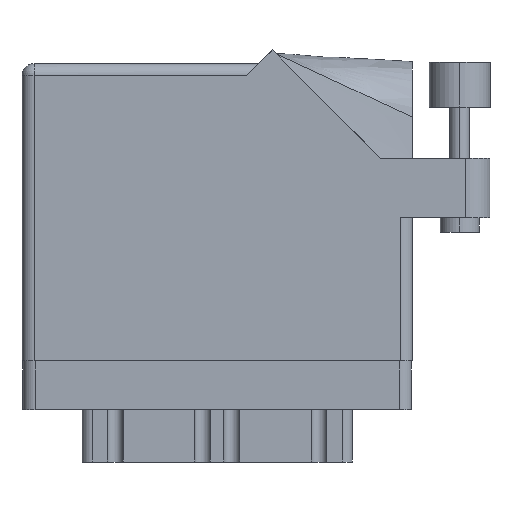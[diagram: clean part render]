
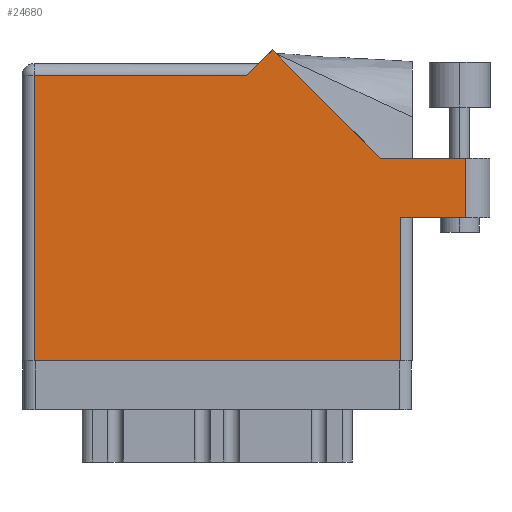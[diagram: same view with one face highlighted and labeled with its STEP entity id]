
A CAD part, front view. The second image highlights one B-rep face of the part: STEP entity #24680.
In plain terms, the highlighted face is planar.
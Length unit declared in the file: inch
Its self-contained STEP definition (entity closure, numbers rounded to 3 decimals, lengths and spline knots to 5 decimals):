
#1559 = ORIENTED_EDGE ( 'NONE', *, *, #2571, .T. ) ;
#2333 = ORIENTED_EDGE ( 'NONE', *, *, #17086, .T. ) ;
#2571 = EDGE_CURVE ( 'NONE', #23713, #5768, #15091, .T. ) ;
#3127 = CARTESIAN_POINT ( 'NONE',  ( 0., 0., 0. ) ) ;
#3396 = EDGE_CURVE ( 'NONE', #16580, #17443, #18091, .T. ) ;
#3887 = VERTEX_POINT ( 'NONE', #12152 ) ;
#4349 = VERTEX_POINT ( 'NONE', #8988 ) ;
#4806 = VECTOR ( 'NONE', #21428, 39.37008 ) ;
#4832 = DIRECTION ( 'NONE',  ( -0.707, -0.707, 0. ) ) ;
#4907 = VECTOR ( 'NONE', #36426, 39.37008 ) ;
#4942 = CARTESIAN_POINT ( 'NONE',  ( 1.948, 0.737, 0. ) ) ;
#5768 = VERTEX_POINT ( 'NONE', #22979 ) ;
#5794 = VECTOR ( 'NONE', #35660, 39.37008 ) ;
#6322 = CARTESIAN_POINT ( 'NONE',  ( 1.84442, 1.044, 0. ) ) ;
#6960 = VECTOR ( 'NONE', #11579, 39.37008 ) ;
#7881 = LINE ( 'NONE', #4942, #11786 ) ;
#8988 = CARTESIAN_POINT ( 'NONE',  ( 0.062, 0., 0. ) ) ;
#9428 = ORIENTED_EDGE ( 'NONE', *, *, #17477, .T. ) ;
#9604 = LINE ( 'NONE', #10342, #4907 ) ;
#9712 = CARTESIAN_POINT ( 'NONE',  ( 1.28771, 1.60071, 0. ) ) ;
#9888 = LINE ( 'NONE', #21854, #22098 ) ;
#10342 = CARTESIAN_POINT ( 'NONE',  ( 2.41, 1.044, 0. ) ) ;
#10674 = CARTESIAN_POINT ( 'NONE',  ( 2.285, 0.737, 0. ) ) ;
#10736 = CARTESIAN_POINT ( 'NONE',  ( 1.217, 1.53, 0. ) ) ;
#10781 = DIRECTION ( 'NONE',  ( 0., 0., -1. ) ) ;
#11579 = DIRECTION ( 'NONE',  ( 0., -1., 0. ) ) ;
#11753 = CARTESIAN_POINT ( 'NONE',  ( 2.285, 1.044, 0. ) ) ;
#11786 = VECTOR ( 'NONE', #23551, 39.37008 ) ;
#12051 = CARTESIAN_POINT ( 'NONE',  ( 1.155, 1.468, 0. ) ) ;
#12087 = ORIENTED_EDGE ( 'NONE', *, *, #24741, .T. ) ;
#12152 = CARTESIAN_POINT ( 'NONE',  ( 1.948, 0.737, 0. ) ) ;
#13011 = DIRECTION ( 'NONE',  ( 1., 0., 0. ) ) ;
#13699 = PLANE ( 'NONE',  #29612 ) ;
#13916 = EDGE_LOOP ( 'NONE', ( #12087, #1559, #15913, #26260, #2333, #9428, #22366, #23523, #27775 ) ) ;
#14127 = LINE ( 'NONE', #31249, #6960 ) ;
#15091 = LINE ( 'NONE', #11753, #26869 ) ;
#15913 = ORIENTED_EDGE ( 'NONE', *, *, #21075, .T. ) ;
#16580 = VERTEX_POINT ( 'NONE', #24160 ) ;
#17086 = EDGE_CURVE ( 'NONE', #17443, #24597, #34630, .T. ) ;
#17443 = VERTEX_POINT ( 'NONE', #9712 ) ;
#17477 = EDGE_CURVE ( 'NONE', #24597, #22713, #30083, .T. ) ;
#18091 = LINE ( 'NONE', #6322, #4806 ) ;
#18712 = CARTESIAN_POINT ( 'NONE',  ( 0., 1.468, 0. ) ) ;
#21075 = EDGE_CURVE ( 'NONE', #5768, #16580, #9604, .T. ) ;
#21428 = DIRECTION ( 'NONE',  ( -0.707, 0.707, 0. ) ) ;
#21854 = CARTESIAN_POINT ( 'NONE',  ( 2.01, 0.737, 0. ) ) ;
#22098 = VECTOR ( 'NONE', #13011, 39.37008 ) ;
#22292 = CARTESIAN_POINT ( 'NONE',  ( 1.948, 0., 0. ) ) ;
#22366 = ORIENTED_EDGE ( 'NONE', *, *, #30171, .T. ) ;
#22713 = VERTEX_POINT ( 'NONE', #32693 ) ;
#22979 = CARTESIAN_POINT ( 'NONE',  ( 2.285, 1.044, 0. ) ) ;
#23523 = ORIENTED_EDGE ( 'NONE', *, *, #24345, .T. ) ;
#23551 = DIRECTION ( 'NONE',  ( 0., 1., 0. ) ) ;
#23713 = VERTEX_POINT ( 'NONE', #10674 ) ;
#24160 = CARTESIAN_POINT ( 'NONE',  ( 1.84442, 1.044, 0. ) ) ;
#24345 = EDGE_CURVE ( 'NONE', #4349, #29642, #32726, .T. ) ;
#24597 = VERTEX_POINT ( 'NONE', #12051 ) ;
#24680 = ADVANCED_FACE ( 'NONE', ( #28605 ), #13699, .F. ) ;
#24741 = EDGE_CURVE ( 'NONE', #3887, #23713, #9888, .T. ) ;
#26260 = ORIENTED_EDGE ( 'NONE', *, *, #3396, .T. ) ;
#26869 = VECTOR ( 'NONE', #35292, 39.37008 ) ;
#26994 = VECTOR ( 'NONE', #4832, 39.37008 ) ;
#27775 = ORIENTED_EDGE ( 'NONE', *, *, #36889, .T. ) ;
#28605 = FACE_OUTER_BOUND ( 'NONE', #13916, .T. ) ;
#29612 = AXIS2_PLACEMENT_3D ( 'NONE', #37588, #10781, #34678 ) ;
#29642 = VERTEX_POINT ( 'NONE', #22292 ) ;
#30083 = LINE ( 'NONE', #18712, #32658 ) ;
#30171 = EDGE_CURVE ( 'NONE', #22713, #4349, #14127, .T. ) ;
#30664 = DIRECTION ( 'NONE',  ( -1., 0., 0. ) ) ;
#31249 = CARTESIAN_POINT ( 'NONE',  ( 0.062, 0., 0. ) ) ;
#32658 = VECTOR ( 'NONE', #30664, 39.37008 ) ;
#32693 = CARTESIAN_POINT ( 'NONE',  ( 0.062, 1.468, 0. ) ) ;
#32726 = LINE ( 'NONE', #3127, #5794 ) ;
#34630 = LINE ( 'NONE', #10736, #26994 ) ;
#34678 = DIRECTION ( 'NONE',  ( -1., 0., 0. ) ) ;
#35292 = DIRECTION ( 'NONE',  ( 0., 1., 0. ) ) ;
#35660 = DIRECTION ( 'NONE',  ( 1., 0., 0. ) ) ;
#36426 = DIRECTION ( 'NONE',  ( -1., 0., 0. ) ) ;
#36889 = EDGE_CURVE ( 'NONE', #29642, #3887, #7881, .T. ) ;
#37588 = CARTESIAN_POINT ( 'NONE',  ( 0., 1.53, 0. ) ) ;
